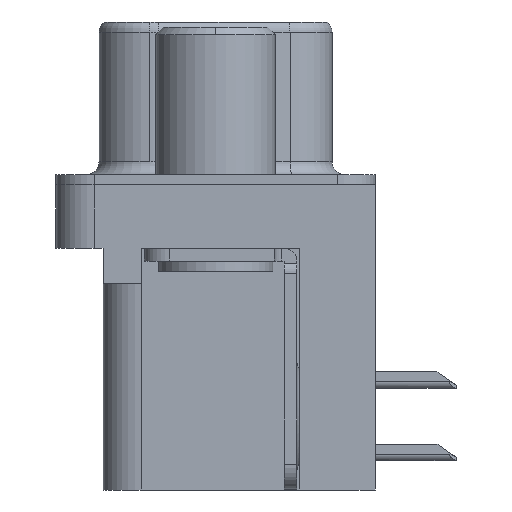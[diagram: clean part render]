
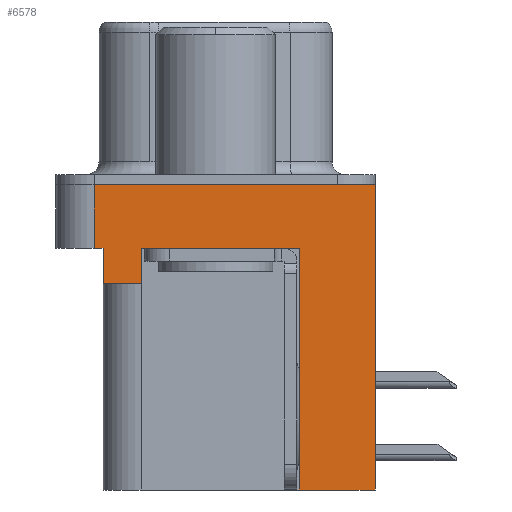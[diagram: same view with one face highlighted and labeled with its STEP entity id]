
A CAD part, left-side view. The second image highlights one B-rep face of the part: STEP entity #6578.
In plain terms, the highlighted planar face has unit normal (-1, 0, 0).
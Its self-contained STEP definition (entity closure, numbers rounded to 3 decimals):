
#14 = DIRECTION ( 'NONE',  ( 0., 0., 1. ) ) ;
#32 = VECTOR ( 'NONE', #15860, 1000. ) ;
#117 = CARTESIAN_POINT ( 'NONE',  ( -2.91, -6.275, -2.5 ) ) ;
#793 = VECTOR ( 'NONE', #9990, 1000. ) ;
#1161 = LINE ( 'NONE', #5999, #32 ) ;
#1232 = LINE ( 'NONE', #3023, #793 ) ;
#2065 = LINE ( 'NONE', #117, #16572 ) ;
#2313 = LINE ( 'NONE', #9676, #16815 ) ;
#2356 = EDGE_CURVE ( 'NONE', #3677, #11886, #1161, .T. ) ;
#2453 = CARTESIAN_POINT ( 'NONE',  ( -2.91, -6.275, 0. ) ) ;
#3023 = CARTESIAN_POINT ( 'NONE',  ( -2.91, -6.275, 0. ) ) ;
#3285 = ORIENTED_EDGE ( 'NONE', *, *, #10892, .F. ) ;
#3341 = LINE ( 'NONE', #14587, #17840 ) ;
#3353 = EDGE_CURVE ( 'NONE', #3918, #10756, #4929, .T. ) ;
#3532 = DIRECTION ( 'NONE',  ( -1., 0., 0. ) ) ;
#3677 = VERTEX_POINT ( 'NONE', #6377 ) ;
#3841 = CARTESIAN_POINT ( 'NONE',  ( -2.91, -3.295, -2.5 ) ) ;
#3866 = VECTOR ( 'NONE', #7988, 1000. ) ;
#3918 = VERTEX_POINT ( 'NONE', #6425 ) ;
#4276 = VERTEX_POINT ( 'NONE', #4802 ) ;
#4710 = CARTESIAN_POINT ( 'NONE',  ( -2.91, -6.275, -2.5 ) ) ;
#4802 = CARTESIAN_POINT ( 'NONE',  ( -2.91, 2.895, -3.9 ) ) ;
#4896 = DIRECTION ( 'NONE',  ( 0., 0., 1. ) ) ;
#4923 = VERTEX_POINT ( 'NONE', #3841 ) ;
#4929 = LINE ( 'NONE', #16884, #11737 ) ;
#5281 = CARTESIAN_POINT ( 'NONE',  ( -2.91, 4.775, -2.5 ) ) ;
#5366 = VECTOR ( 'NONE', #7545, 1000. ) ;
#5750 = VECTOR ( 'NONE', #12001, 1000. ) ;
#5999 = CARTESIAN_POINT ( 'NONE',  ( -2.91, -3.295, -12. ) ) ;
#6131 = PLANE ( 'NONE',  #7338 ) ;
#6377 = CARTESIAN_POINT ( 'NONE',  ( -2.91, -6.275, -12. ) ) ;
#6425 = CARTESIAN_POINT ( 'NONE',  ( -2.91, 4.775, -2.5 ) ) ;
#6460 = EDGE_CURVE ( 'NONE', #12553, #6859, #1232, .T. ) ;
#6578 = ADVANCED_FACE ( 'NONE', ( #8968 ), #6131, .T. ) ;
#6706 = ORIENTED_EDGE ( 'NONE', *, *, #11979, .T. ) ;
#6721 = CARTESIAN_POINT ( 'NONE',  ( -2.91, 4.425, -3.9 ) ) ;
#6859 = VERTEX_POINT ( 'NONE', #2453 ) ;
#7338 = AXIS2_PLACEMENT_3D ( 'NONE', #4710, #3532, #4896 ) ;
#7545 = DIRECTION ( 'NONE',  ( 0., 0., 1. ) ) ;
#7680 = VECTOR ( 'NONE', #9502, 1000. ) ;
#7988 = DIRECTION ( 'NONE',  ( 0., 0., 1. ) ) ;
#8623 = EDGE_CURVE ( 'NONE', #4276, #14298, #15507, .T. ) ;
#8804 = ORIENTED_EDGE ( 'NONE', *, *, #3353, .T. ) ;
#8968 = FACE_OUTER_BOUND ( 'NONE', #16834, .T. ) ;
#9180 = CARTESIAN_POINT ( 'NONE',  ( -2.91, -6.275, -2.5 ) ) ;
#9198 = EDGE_CURVE ( 'NONE', #3677, #6859, #2065, .T. ) ;
#9502 = DIRECTION ( 'NONE',  ( 0., 0., 1. ) ) ;
#9676 = CARTESIAN_POINT ( 'NONE',  ( -2.91, -3.295, -12. ) ) ;
#9990 = DIRECTION ( 'NONE',  ( 0., -1., 0. ) ) ;
#10197 = DIRECTION ( 'NONE',  ( 0., 0., 1. ) ) ;
#10204 = EDGE_CURVE ( 'NONE', #15959, #10756, #12610, .T. ) ;
#10297 = CARTESIAN_POINT ( 'NONE',  ( -2.91, 4.425, -2.5 ) ) ;
#10502 = CARTESIAN_POINT ( 'NONE',  ( -2.91, 4.425, -3.9 ) ) ;
#10548 = DIRECTION ( 'NONE',  ( 0., 1., 0. ) ) ;
#10756 = VERTEX_POINT ( 'NONE', #10297 ) ;
#10892 = EDGE_CURVE ( 'NONE', #4276, #15959, #3341, .T. ) ;
#11273 = ORIENTED_EDGE ( 'NONE', *, *, #6460, .F. ) ;
#11632 = LINE ( 'NONE', #5281, #7680 ) ;
#11737 = VECTOR ( 'NONE', #15846, 1000. ) ;
#11886 = VERTEX_POINT ( 'NONE', #17744 ) ;
#11979 = EDGE_CURVE ( 'NONE', #14298, #4923, #15203, .T. ) ;
#12001 = DIRECTION ( 'NONE',  ( 0., -1., 0. ) ) ;
#12377 = ORIENTED_EDGE ( 'NONE', *, *, #9198, .T. ) ;
#12553 = VERTEX_POINT ( 'NONE', #13753 ) ;
#12610 = LINE ( 'NONE', #10502, #5366 ) ;
#13753 = CARTESIAN_POINT ( 'NONE',  ( -2.91, 4.775, 0. ) ) ;
#13878 = ORIENTED_EDGE ( 'NONE', *, *, #10204, .F. ) ;
#14298 = VERTEX_POINT ( 'NONE', #14735 ) ;
#14587 = CARTESIAN_POINT ( 'NONE',  ( -2.91, 4.425, -3.9 ) ) ;
#14666 = ORIENTED_EDGE ( 'NONE', *, *, #15254, .F. ) ;
#14735 = CARTESIAN_POINT ( 'NONE',  ( -2.91, 2.895, -2.5 ) ) ;
#15203 = LINE ( 'NONE', #9180, #5750 ) ;
#15254 = EDGE_CURVE ( 'NONE', #11886, #4923, #2313, .T. ) ;
#15507 = LINE ( 'NONE', #17726, #3866 ) ;
#15693 = ORIENTED_EDGE ( 'NONE', *, *, #2356, .F. ) ;
#15846 = DIRECTION ( 'NONE',  ( 0., -1., 0. ) ) ;
#15860 = DIRECTION ( 'NONE',  ( 0., 1., 0. ) ) ;
#15959 = VERTEX_POINT ( 'NONE', #6721 ) ;
#16572 = VECTOR ( 'NONE', #10197, 1000. ) ;
#16679 = ORIENTED_EDGE ( 'NONE', *, *, #17299, .F. ) ;
#16815 = VECTOR ( 'NONE', #14, 1000. ) ;
#16834 = EDGE_LOOP ( 'NONE', ( #11273, #16679, #8804, #13878, #3285, #17327, #6706, #14666, #15693, #12377 ) ) ;
#16884 = CARTESIAN_POINT ( 'NONE',  ( -2.91, -6.275, -2.5 ) ) ;
#17299 = EDGE_CURVE ( 'NONE', #3918, #12553, #11632, .T. ) ;
#17327 = ORIENTED_EDGE ( 'NONE', *, *, #8623, .T. ) ;
#17726 = CARTESIAN_POINT ( 'NONE',  ( -2.91, 2.895, -3.9 ) ) ;
#17744 = CARTESIAN_POINT ( 'NONE',  ( -2.91, -3.295, -12. ) ) ;
#17840 = VECTOR ( 'NONE', #10548, 1000. ) ;
